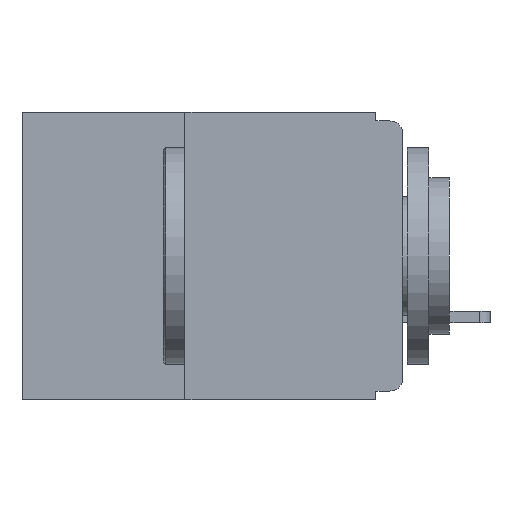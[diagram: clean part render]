
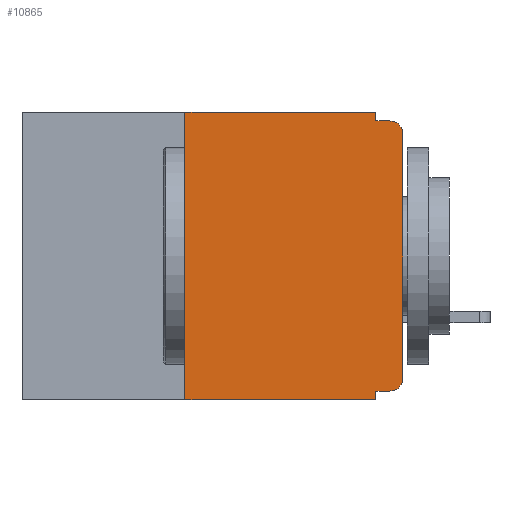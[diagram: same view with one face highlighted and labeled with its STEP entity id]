
A CAD part, left-side view. The second image highlights one B-rep face of the part: STEP entity #10865.
In plain terms, the highlighted planar face has unit normal (-1, 0, 0).
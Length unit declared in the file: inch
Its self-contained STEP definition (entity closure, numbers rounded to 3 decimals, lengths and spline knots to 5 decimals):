
#60 = LINE ( 'NONE', #18117, #18698 ) ;
#273 = VERTEX_POINT ( 'NONE', #10944 ) ;
#401 = VERTEX_POINT ( 'NONE', #763 ) ;
#688 = DIRECTION ( 'NONE',  ( 0., 0., -1. ) ) ;
#754 = EDGE_LOOP ( 'NONE', ( #20995, #21521, #21606, #12360, #8772, #12969, #6770, #9424, #2598, #14246 ) ) ;
#763 = CARTESIAN_POINT ( 'NONE',  ( 0., 0.031, -0.33 ) ) ;
#812 = DIRECTION ( 'NONE',  ( 0., -1., 0. ) ) ;
#833 = DIRECTION ( 'NONE',  ( -1., 0., 0. ) ) ;
#1101 = VERTEX_POINT ( 'NONE', #23265 ) ;
#2231 = LINE ( 'NONE', #15994, #13302 ) ;
#2598 = ORIENTED_EDGE ( 'NONE', *, *, #9486, .F. ) ;
#2877 = LINE ( 'NONE', #13889, #11986 ) ;
#3264 = LINE ( 'NONE', #18905, #20807 ) ;
#3496 = CARTESIAN_POINT ( 'NONE',  ( 0., 0.031, -0.33 ) ) ;
#3703 = CARTESIAN_POINT ( 'NONE',  ( 0., 0.437, 0. ) ) ;
#3767 = DIRECTION ( 'NONE',  ( 0., 0., 1. ) ) ;
#3975 = VECTOR ( 'NONE', #15861, 39.37008 ) ;
#4135 = EDGE_CURVE ( 'NONE', #23264, #401, #9476, .T. ) ;
#4432 = LINE ( 'NONE', #18781, #13526 ) ;
#4434 = CARTESIAN_POINT ( 'NONE',  ( 0., 0.031, -0.32 ) ) ;
#4838 = DIRECTION ( 'NONE',  ( 0., -1., 0. ) ) ;
#5004 = VERTEX_POINT ( 'NONE', #16032 ) ;
#5542 = DIRECTION ( 'NONE',  ( 1., 0., 0. ) ) ;
#5797 = EDGE_CURVE ( 'NONE', #21614, #8391, #2877, .T. ) ;
#6184 = VERTEX_POINT ( 'NONE', #4434 ) ;
#6770 = ORIENTED_EDGE ( 'NONE', *, *, #4135, .T. ) ;
#7381 = EDGE_CURVE ( 'NONE', #273, #5004, #14830, .T. ) ;
#7899 = AXIS2_PLACEMENT_3D ( 'NONE', #8811, #21468, #10654 ) ;
#8242 = DIRECTION ( 'NONE',  ( 0., -1., 0. ) ) ;
#8268 = CARTESIAN_POINT ( 'NONE',  ( 0., 0., 0. ) ) ;
#8321 = CARTESIAN_POINT ( 'NONE',  ( 0., 0.437, -0.33 ) ) ;
#8377 = EDGE_CURVE ( 'NONE', #6184, #401, #23190, .T. ) ;
#8391 = VERTEX_POINT ( 'NONE', #14455 ) ;
#8772 = ORIENTED_EDGE ( 'NONE', *, *, #5797, .F. ) ;
#8811 = CARTESIAN_POINT ( 'NONE',  ( 0., 0.015, -0.305 ) ) ;
#8903 = VECTOR ( 'NONE', #8242, 39.37008 ) ;
#9131 = VECTOR ( 'NONE', #15524, 39.37008 ) ;
#9424 = ORIENTED_EDGE ( 'NONE', *, *, #8377, .F. ) ;
#9476 = LINE ( 'NONE', #8321, #8903 ) ;
#9486 = EDGE_CURVE ( 'NONE', #11048, #6184, #2231, .T. ) ;
#9699 = LINE ( 'NONE', #8268, #9131 ) ;
#10161 = EDGE_CURVE ( 'NONE', #11048, #23383, #22004, .T. ) ;
#10654 = DIRECTION ( 'NONE',  ( 0., 0., -1. ) ) ;
#10865 = ADVANCED_FACE ( 'NONE', ( #16348 ), #14588, .F. ) ;
#10944 = CARTESIAN_POINT ( 'NONE',  ( 0., 0., -0.025 ) ) ;
#11048 = VERTEX_POINT ( 'NONE', #13235 ) ;
#11398 = CARTESIAN_POINT ( 'NONE',  ( 0., 0.25, 0. ) ) ;
#11408 = AXIS2_PLACEMENT_3D ( 'NONE', #3703, #5542, #18216 ) ;
#11670 = CARTESIAN_POINT ( 'NONE',  ( 0., 0.015, -0.025 ) ) ;
#11986 = VECTOR ( 'NONE', #4838, 39.37008 ) ;
#12360 = ORIENTED_EDGE ( 'NONE', *, *, #19227, .F. ) ;
#12969 = ORIENTED_EDGE ( 'NONE', *, *, #14595, .F. ) ;
#13235 = CARTESIAN_POINT ( 'NONE',  ( 0., 0.015, -0.32 ) ) ;
#13302 = VECTOR ( 'NONE', #17794, 39.37008 ) ;
#13508 = DIRECTION ( 'NONE',  ( 0., 0., -1. ) ) ;
#13526 = VECTOR ( 'NONE', #688, 39.37008 ) ;
#13889 = CARTESIAN_POINT ( 'NONE',  ( 0., 0.437, 0. ) ) ;
#14246 = ORIENTED_EDGE ( 'NONE', *, *, #10161, .T. ) ;
#14330 = CARTESIAN_POINT ( 'NONE',  ( 0., 0.25, -0.33 ) ) ;
#14455 = CARTESIAN_POINT ( 'NONE',  ( 0., 0.031, 0. ) ) ;
#14588 = PLANE ( 'NONE',  #11408 ) ;
#14595 = EDGE_CURVE ( 'NONE', #23264, #21614, #60, .T. ) ;
#14643 = CARTESIAN_POINT ( 'NONE',  ( 0., 0., -0.305 ) ) ;
#14830 = CIRCLE ( 'NONE', #19684, 0.015 ) ;
#15524 = DIRECTION ( 'NONE',  ( 0., 0., 1. ) ) ;
#15861 = DIRECTION ( 'NONE',  ( 0., 0., -1. ) ) ;
#15994 = CARTESIAN_POINT ( 'NONE',  ( 0., 0., -0.32 ) ) ;
#16032 = CARTESIAN_POINT ( 'NONE',  ( 0., 0.015, -0.01 ) ) ;
#16348 = FACE_OUTER_BOUND ( 'NONE', #754, .T. ) ;
#17794 = DIRECTION ( 'NONE',  ( 0., 1., 0. ) ) ;
#18117 = CARTESIAN_POINT ( 'NONE',  ( 0., 0.25, -0.33 ) ) ;
#18140 = EDGE_CURVE ( 'NONE', #1101, #5004, #3264, .T. ) ;
#18216 = DIRECTION ( 'NONE',  ( 0., 0., -1. ) ) ;
#18698 = VECTOR ( 'NONE', #3767, 39.37008 ) ;
#18781 = CARTESIAN_POINT ( 'NONE',  ( 0., 0.031, 0. ) ) ;
#18905 = CARTESIAN_POINT ( 'NONE',  ( 0., 0., -0.01 ) ) ;
#19227 = EDGE_CURVE ( 'NONE', #8391, #1101, #4432, .T. ) ;
#19684 = AXIS2_PLACEMENT_3D ( 'NONE', #11670, #833, #13508 ) ;
#20807 = VECTOR ( 'NONE', #812, 39.37008 ) ;
#20995 = ORIENTED_EDGE ( 'NONE', *, *, #21788, .T. ) ;
#21468 = DIRECTION ( 'NONE',  ( -1., 0., 0. ) ) ;
#21521 = ORIENTED_EDGE ( 'NONE', *, *, #7381, .T. ) ;
#21606 = ORIENTED_EDGE ( 'NONE', *, *, #18140, .F. ) ;
#21614 = VERTEX_POINT ( 'NONE', #11398 ) ;
#21788 = EDGE_CURVE ( 'NONE', #23383, #273, #9699, .T. ) ;
#22004 = CIRCLE ( 'NONE', #7899, 0.015 ) ;
#23190 = LINE ( 'NONE', #3496, #3975 ) ;
#23264 = VERTEX_POINT ( 'NONE', #14330 ) ;
#23265 = CARTESIAN_POINT ( 'NONE',  ( 0., 0.031, -0.01 ) ) ;
#23383 = VERTEX_POINT ( 'NONE', #14643 ) ;
